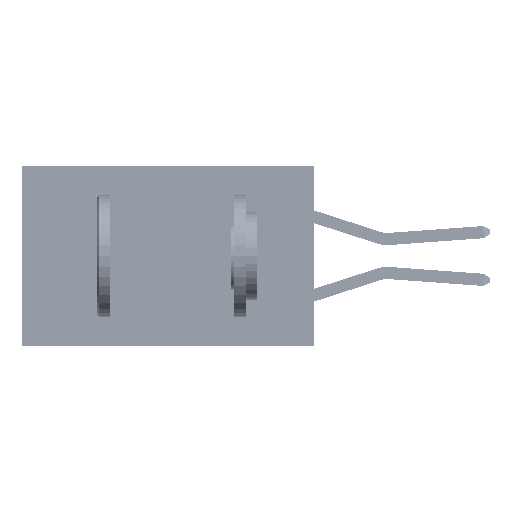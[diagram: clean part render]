
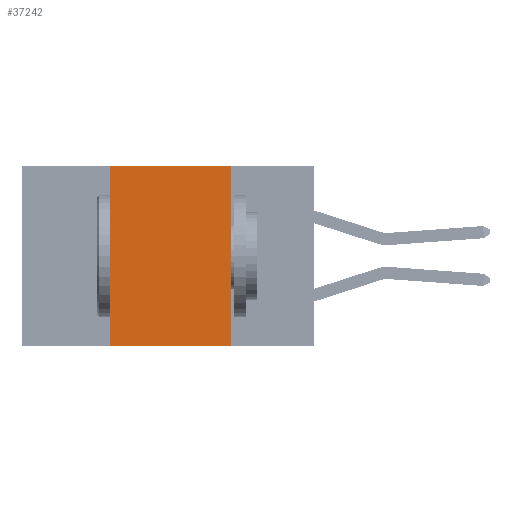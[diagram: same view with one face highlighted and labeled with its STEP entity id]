
A CAD part, left-side view. The second image highlights one B-rep face of the part: STEP entity #37242.
In plain terms, the highlighted planar face has unit normal (-1, 0, 0).
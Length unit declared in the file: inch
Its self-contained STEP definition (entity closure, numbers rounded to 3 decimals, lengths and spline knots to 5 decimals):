
#1206 = VECTOR ( 'NONE', #48248, 39.37008 ) ;
#1586 = EDGE_CURVE ( 'NONE', #10245, #16733, #28968, .T. ) ;
#1636 = ORIENTED_EDGE ( 'NONE', *, *, #20347, .T. ) ;
#3608 = CARTESIAN_POINT ( 'NONE',  ( 0., 0.42, 0. ) ) ;
#6431 = DIRECTION ( 'NONE',  ( 0., 0., -1. ) ) ;
#7303 = CARTESIAN_POINT ( 'NONE',  ( 0., 0.6, 0. ) ) ;
#10245 = VERTEX_POINT ( 'NONE', #24566 ) ;
#12702 = EDGE_LOOP ( 'NONE', ( #50237, #33651, #14414, #1636 ) ) ;
#14414 = ORIENTED_EDGE ( 'NONE', *, *, #1586, .F. ) ;
#16733 = VERTEX_POINT ( 'NONE', #22753 ) ;
#18376 = CARTESIAN_POINT ( 'NONE',  ( 0., 0.6, 0. ) ) ;
#19291 = DIRECTION ( 'NONE',  ( 1., 0., 0. ) ) ;
#19538 = CARTESIAN_POINT ( 'NONE',  ( 0., 0.17, 0. ) ) ;
#20347 = EDGE_CURVE ( 'NONE', #10245, #30565, #22445, .T. ) ;
#20399 = CARTESIAN_POINT ( 'NONE',  ( 0., 0.6, -0.37 ) ) ;
#22445 = LINE ( 'NONE', #20399, #1206 ) ;
#22753 = CARTESIAN_POINT ( 'NONE',  ( 0., 0.42, 0. ) ) ;
#24566 = CARTESIAN_POINT ( 'NONE',  ( 0., 0.42, -0.37 ) ) ;
#25757 = VERTEX_POINT ( 'NONE', #19538 ) ;
#25853 = LINE ( 'NONE', #41952, #35176 ) ;
#27066 = PLANE ( 'NONE',  #33337 ) ;
#28968 = LINE ( 'NONE', #3608, #48778 ) ;
#30565 = VERTEX_POINT ( 'NONE', #47600 ) ;
#33337 = AXIS2_PLACEMENT_3D ( 'NONE', #7303, #19291, #46984 ) ;
#33651 = ORIENTED_EDGE ( 'NONE', *, *, #42945, .F. ) ;
#35176 = VECTOR ( 'NONE', #6431, 39.37008 ) ;
#37242 = ADVANCED_FACE ( 'NONE', ( #45485 ), #27066, .F. ) ;
#39878 = EDGE_CURVE ( 'NONE', #25757, #30565, #25853, .T. ) ;
#41952 = CARTESIAN_POINT ( 'NONE',  ( 0., 0.17, 0. ) ) ;
#42099 = DIRECTION ( 'NONE',  ( 0., -1., 0. ) ) ;
#42945 = EDGE_CURVE ( 'NONE', #16733, #25757, #47827, .T. ) ;
#45485 = FACE_OUTER_BOUND ( 'NONE', #12702, .T. ) ;
#46589 = VECTOR ( 'NONE', #42099, 39.37008 ) ;
#46984 = DIRECTION ( 'NONE',  ( 0., 0., -1. ) ) ;
#47344 = DIRECTION ( 'NONE',  ( 0., 0., 1. ) ) ;
#47600 = CARTESIAN_POINT ( 'NONE',  ( 0., 0.17, -0.37 ) ) ;
#47827 = LINE ( 'NONE', #18376, #46589 ) ;
#48248 = DIRECTION ( 'NONE',  ( 0., -1., 0. ) ) ;
#48778 = VECTOR ( 'NONE', #47344, 39.37008 ) ;
#50237 = ORIENTED_EDGE ( 'NONE', *, *, #39878, .F. ) ;
